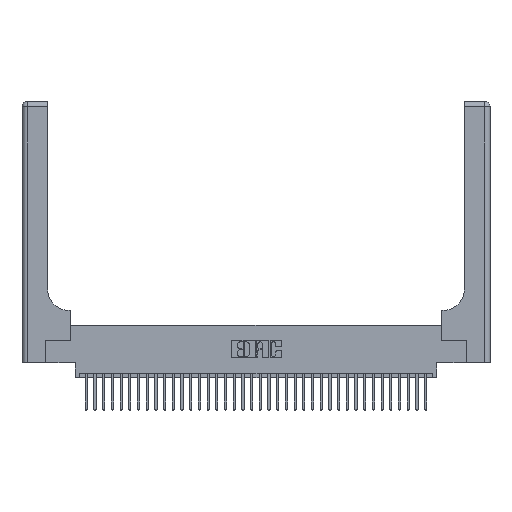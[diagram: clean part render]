
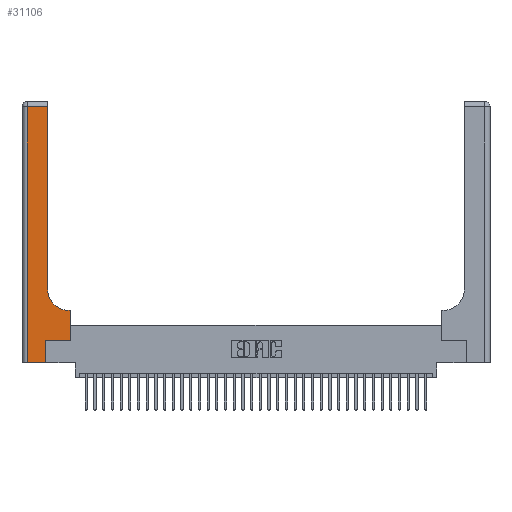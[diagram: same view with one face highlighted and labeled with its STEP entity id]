
A CAD part, top view. The second image highlights one B-rep face of the part: STEP entity #31106.
In plain terms, the highlighted planar face has unit normal (0, 0, 1).
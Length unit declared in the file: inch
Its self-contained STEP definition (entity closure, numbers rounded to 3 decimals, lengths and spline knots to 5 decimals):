
#383 = CARTESIAN_POINT ( 'NONE',  ( 0.2915, 0.6, 0.37 ) ) ;
#909 = LINE ( 'NONE', #383, #9384 ) ;
#1207 = DIRECTION ( 'NONE',  ( 0., 1., 0. ) ) ;
#1728 = CARTESIAN_POINT ( 'NONE',  ( 0.269, 0.25, 0.37 ) ) ;
#2568 = CARTESIAN_POINT ( 'NONE',  ( 0.06, 0., 0.37 ) ) ;
#4184 = CARTESIAN_POINT ( 'NONE',  ( 0.269, 0., 0.37 ) ) ;
#4597 = CARTESIAN_POINT ( 'NONE',  ( 0.5585, 0.25, 0.37 ) ) ;
#5095 = DIRECTION ( 'NONE',  ( 0., 1., 0. ) ) ;
#5334 = CARTESIAN_POINT ( 'NONE',  ( 0., 3., 0.37 ) ) ;
#5514 = VECTOR ( 'NONE', #19744, 39.37008 ) ;
#6253 = VERTEX_POINT ( 'NONE', #2568 ) ;
#6849 = CARTESIAN_POINT ( 'NONE',  ( 0.2915, 2.94, 0.37 ) ) ;
#7162 = EDGE_CURVE ( 'NONE', #34907, #34910, #24340, .T. ) ;
#8174 = VECTOR ( 'NONE', #9365, 39.37008 ) ;
#8200 = DIRECTION ( 'NONE',  ( -1., 0., 0. ) ) ;
#9147 = VERTEX_POINT ( 'NONE', #14545 ) ;
#9365 = DIRECTION ( 'NONE',  ( 1., 0., 0. ) ) ;
#9384 = VECTOR ( 'NONE', #20552, 39.37008 ) ;
#9711 = CARTESIAN_POINT ( 'NONE',  ( 0.5415, 0.6, 0.37 ) ) ;
#9716 = ORIENTED_EDGE ( 'NONE', *, *, #31482, .T. ) ;
#9756 = ORIENTED_EDGE ( 'NONE', *, *, #10892, .T. ) ;
#9895 = ORIENTED_EDGE ( 'NONE', *, *, #27963, .T. ) ;
#10892 = EDGE_CURVE ( 'NONE', #9147, #30799, #909, .T. ) ;
#11041 = DIRECTION ( 'NONE',  ( 0., 0., -1. ) ) ;
#11292 = DIRECTION ( 'NONE',  ( 1., 0., 0. ) ) ;
#12326 = LINE ( 'NONE', #19390, #26679 ) ;
#12515 = LINE ( 'NONE', #25566, #26862 ) ;
#13126 = LINE ( 'NONE', #36817, #5514 ) ;
#13565 = CARTESIAN_POINT ( 'NONE',  ( 0.2915, 0.85, 0.37 ) ) ;
#14159 = CARTESIAN_POINT ( 'NONE',  ( 0.2915, 3., 0.37 ) ) ;
#14290 = DIRECTION ( 'NONE',  ( 0., 1., 0. ) ) ;
#14545 = CARTESIAN_POINT ( 'NONE',  ( 0.5585, 0.6, 0.37 ) ) ;
#15784 = EDGE_CURVE ( 'NONE', #34910, #9147, #12326, .T. ) ;
#16901 = VECTOR ( 'NONE', #14290, 39.37008 ) ;
#17004 = CARTESIAN_POINT ( 'NONE',  ( 0.06, 2.94, 0.37 ) ) ;
#17798 = LINE ( 'NONE', #14159, #16901 ) ;
#18315 = CARTESIAN_POINT ( 'NONE',  ( 0., 2.94, 0.37 ) ) ;
#18593 = VECTOR ( 'NONE', #21237, 39.37008 ) ;
#19390 = CARTESIAN_POINT ( 'NONE',  ( 0.5585, 0.25, 0.37 ) ) ;
#19744 = DIRECTION ( 'NONE',  ( 0., -1., 0. ) ) ;
#20552 = DIRECTION ( 'NONE',  ( -1., 0., 0. ) ) ;
#20906 = VERTEX_POINT ( 'NONE', #6849 ) ;
#21237 = DIRECTION ( 'NONE',  ( -1., 0., 0. ) ) ;
#21291 = EDGE_LOOP ( 'NONE', ( #9895, #32722, #31661, #31230, #9716, #24535, #33936, #9756, #33506 ) ) ;
#22385 = VECTOR ( 'NONE', #1207, 39.37008 ) ;
#22791 = EDGE_CURVE ( 'NONE', #20906, #36484, #26210, .T. ) ;
#24165 = VERTEX_POINT ( 'NONE', #13565 ) ;
#24220 = EDGE_CURVE ( 'NONE', #30799, #24165, #33698, .T. ) ;
#24340 = LINE ( 'NONE', #29418, #8174 ) ;
#24535 = ORIENTED_EDGE ( 'NONE', *, *, #7162, .T. ) ;
#25363 = DIRECTION ( 'NONE',  ( 0., 0., -1. ) ) ;
#25566 = CARTESIAN_POINT ( 'NONE',  ( 0., 0., 0.37 ) ) ;
#26210 = LINE ( 'NONE', #18315, #18593 ) ;
#26429 = FACE_OUTER_BOUND ( 'NONE', #21291, .T. ) ;
#26476 = VERTEX_POINT ( 'NONE', #4184 ) ;
#26679 = VECTOR ( 'NONE', #5095, 39.37008 ) ;
#26744 = EDGE_CURVE ( 'NONE', #6253, #26476, #12515, .T. ) ;
#26862 = VECTOR ( 'NONE', #11292, 39.37008 ) ;
#27963 = EDGE_CURVE ( 'NONE', #24165, #20906, #17798, .T. ) ;
#28129 = PLANE ( 'NONE',  #35351 ) ;
#28208 = CARTESIAN_POINT ( 'NONE',  ( 0.5415, 0.85, 0.37 ) ) ;
#29257 = EDGE_CURVE ( 'NONE', #36484, #6253, #13126, .T. ) ;
#29418 = CARTESIAN_POINT ( 'NONE',  ( 0.269, 0.25, 0.37 ) ) ;
#30799 = VERTEX_POINT ( 'NONE', #9711 ) ;
#30895 = LINE ( 'NONE', #35452, #22385 ) ;
#31106 = ADVANCED_FACE ( 'NONE', ( #26429 ), #28129, .F. ) ;
#31108 = DIRECTION ( 'NONE',  ( 1., 0., 0. ) ) ;
#31230 = ORIENTED_EDGE ( 'NONE', *, *, #26744, .T. ) ;
#31482 = EDGE_CURVE ( 'NONE', #26476, #34907, #30895, .T. ) ;
#31661 = ORIENTED_EDGE ( 'NONE', *, *, #29257, .T. ) ;
#32722 = ORIENTED_EDGE ( 'NONE', *, *, #22791, .T. ) ;
#33506 = ORIENTED_EDGE ( 'NONE', *, *, #24220, .T. ) ;
#33582 = AXIS2_PLACEMENT_3D ( 'NONE', #28208, #11041, #31108 ) ;
#33698 = CIRCLE ( 'NONE', #33582, 0.25 ) ;
#33936 = ORIENTED_EDGE ( 'NONE', *, *, #15784, .T. ) ;
#34907 = VERTEX_POINT ( 'NONE', #1728 ) ;
#34910 = VERTEX_POINT ( 'NONE', #4597 ) ;
#35351 = AXIS2_PLACEMENT_3D ( 'NONE', #5334, #25363, #8200 ) ;
#35452 = CARTESIAN_POINT ( 'NONE',  ( 0.269, 0., 0.37 ) ) ;
#36484 = VERTEX_POINT ( 'NONE', #17004 ) ;
#36817 = CARTESIAN_POINT ( 'NONE',  ( 0.06, 3., 0.37 ) ) ;
